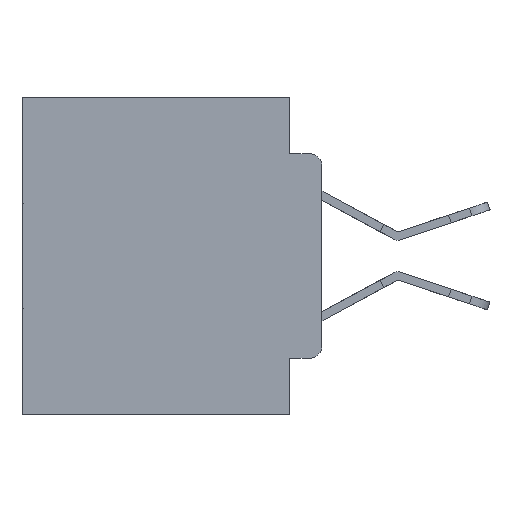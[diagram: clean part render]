
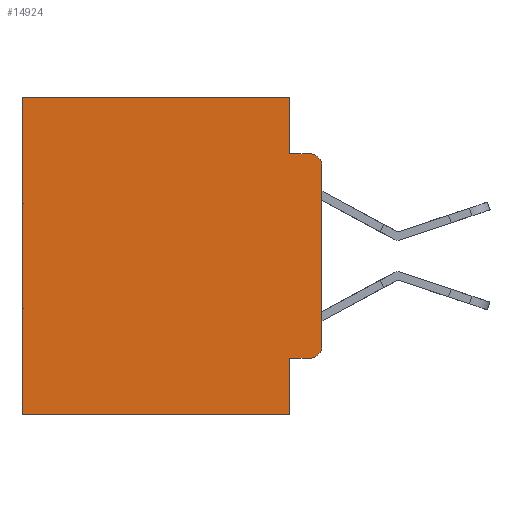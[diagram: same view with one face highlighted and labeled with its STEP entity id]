
A CAD part, left-side view. The second image highlights one B-rep face of the part: STEP entity #14924.
In plain terms, the highlighted planar face has unit normal (-1, 0, 0).
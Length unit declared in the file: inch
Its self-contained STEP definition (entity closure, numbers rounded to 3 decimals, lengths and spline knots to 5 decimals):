
#461 = DIRECTION ( 'NONE',  ( 0., -1., 0. ) ) ;
#847 = ORIENTED_EDGE ( 'NONE', *, *, #24118, .T. ) ;
#1697 = LINE ( 'NONE', #16504, #26920 ) ;
#1742 = LINE ( 'NONE', #30964, #8446 ) ;
#2425 = DIRECTION ( 'NONE',  ( -1., 0., 0. ) ) ;
#3101 = CARTESIAN_POINT ( 'NONE',  ( 0.298, 0., 0. ) ) ;
#3531 = VERTEX_POINT ( 'NONE', #8795 ) ;
#4022 = CARTESIAN_POINT ( 'NONE',  ( 0.298, 0.473, 0. ) ) ;
#4408 = ORIENTED_EDGE ( 'NONE', *, *, #8390, .F. ) ;
#4509 = EDGE_CURVE ( 'NONE', #24833, #29772, #18690, .T. ) ;
#4597 = CARTESIAN_POINT ( 'NONE',  ( 0.298, 0.02, -0.4115 ) ) ;
#4876 = CARTESIAN_POINT ( 'NONE',  ( 0.298, 0.051, 0. ) ) ;
#4918 = LINE ( 'NONE', #25913, #17300 ) ;
#5654 = DIRECTION ( 'NONE',  ( 0., 0., -1. ) ) ;
#5695 = VECTOR ( 'NONE', #27521, 39.37008 ) ;
#6582 = DIRECTION ( 'NONE',  ( 0., 0., -1. ) ) ;
#7586 = ORIENTED_EDGE ( 'NONE', *, *, #30619, .F. ) ;
#8390 = EDGE_CURVE ( 'NONE', #15049, #25976, #20808, .T. ) ;
#8446 = VECTOR ( 'NONE', #16836, 39.37008 ) ;
#8795 = CARTESIAN_POINT ( 'NONE',  ( 0.298, 0.051, -0.4115 ) ) ;
#9903 = ORIENTED_EDGE ( 'NONE', *, *, #19263, .T. ) ;
#9938 = CARTESIAN_POINT ( 'NONE',  ( 0.298, 0.473, -0.5 ) ) ;
#10428 = CARTESIAN_POINT ( 'NONE',  ( 0.298, 0.051, -0.5 ) ) ;
#10739 = VERTEX_POINT ( 'NONE', #20066 ) ;
#10905 = FACE_OUTER_BOUND ( 'NONE', #30051, .T. ) ;
#11100 = AXIS2_PLACEMENT_3D ( 'NONE', #3101, #20354, #5654 ) ;
#11311 = EDGE_CURVE ( 'NONE', #15049, #10739, #18377, .T. ) ;
#11324 = VECTOR ( 'NONE', #461, 39.37008 ) ;
#11823 = ORIENTED_EDGE ( 'NONE', *, *, #30928, .F. ) ;
#12268 = CARTESIAN_POINT ( 'NONE',  ( 0.298, 0.02, -0.3915 ) ) ;
#12626 = ORIENTED_EDGE ( 'NONE', *, *, #4509, .T. ) ;
#13394 = VERTEX_POINT ( 'NONE', #10428 ) ;
#14208 = EDGE_CURVE ( 'NONE', #3531, #27843, #17866, .T. ) ;
#14398 = VECTOR ( 'NONE', #19145, 39.37008 ) ;
#14539 = CARTESIAN_POINT ( 'NONE',  ( 0.298, 0.051, -0.0885 ) ) ;
#14729 = VECTOR ( 'NONE', #6582, 39.37008 ) ;
#14781 = DIRECTION ( 'NONE',  ( 0., 0., -1. ) ) ;
#14924 = ADVANCED_FACE ( 'NONE', ( #10905 ), #17952, .F. ) ;
#15049 = VERTEX_POINT ( 'NONE', #20870 ) ;
#15454 = CARTESIAN_POINT ( 'NONE',  ( 0.298, 0.051, -0.4115 ) ) ;
#15713 = ORIENTED_EDGE ( 'NONE', *, *, #14208, .T. ) ;
#15760 = AXIS2_PLACEMENT_3D ( 'NONE', #12268, #29025, #14781 ) ;
#16504 = CARTESIAN_POINT ( 'NONE',  ( 0.298, 0.051, 0. ) ) ;
#16836 = DIRECTION ( 'NONE',  ( 0., 1., 0. ) ) ;
#17300 = VECTOR ( 'NONE', #21159, 39.37008 ) ;
#17305 = CARTESIAN_POINT ( 'NONE',  ( 0.298, 0.02, -0.1085 ) ) ;
#17590 = ORIENTED_EDGE ( 'NONE', *, *, #11311, .T. ) ;
#17866 = LINE ( 'NONE', #15454, #11324 ) ;
#17952 = PLANE ( 'NONE',  #11100 ) ;
#18350 = ORIENTED_EDGE ( 'NONE', *, *, #30535, .F. ) ;
#18377 = CIRCLE ( 'NONE', #22260, 0.02 ) ;
#18480 = EDGE_CURVE ( 'NONE', #3531, #13394, #1697, .T. ) ;
#18690 = LINE ( 'NONE', #30323, #19447 ) ;
#18784 = LINE ( 'NONE', #22796, #5695 ) ;
#19145 = DIRECTION ( 'NONE',  ( 0., 0., -1. ) ) ;
#19263 = EDGE_CURVE ( 'NONE', #27843, #25976, #29083, .T. ) ;
#19447 = VECTOR ( 'NONE', #25054, 39.37008 ) ;
#19733 = DIRECTION ( 'NONE',  ( 0., 0., -1. ) ) ;
#20066 = CARTESIAN_POINT ( 'NONE',  ( 0.298, 0.02, -0.0885 ) ) ;
#20354 = DIRECTION ( 'NONE',  ( 1., 0., 0. ) ) ;
#20601 = ORIENTED_EDGE ( 'NONE', *, *, #18480, .F. ) ;
#20808 = LINE ( 'NONE', #28567, #14398 ) ;
#20870 = CARTESIAN_POINT ( 'NONE',  ( 0.298, 0., -0.1085 ) ) ;
#21159 = DIRECTION ( 'NONE',  ( 0., 0., -1. ) ) ;
#22260 = AXIS2_PLACEMENT_3D ( 'NONE', #17305, #2425, #19733 ) ;
#22796 = CARTESIAN_POINT ( 'NONE',  ( 0.298, 0.051, -0.0885 ) ) ;
#23073 = CARTESIAN_POINT ( 'NONE',  ( 0.298, 0.473, 0. ) ) ;
#24118 = EDGE_CURVE ( 'NONE', #29772, #30760, #25933, .T. ) ;
#24833 = VERTEX_POINT ( 'NONE', #4876 ) ;
#25054 = DIRECTION ( 'NONE',  ( 0., 1., 0. ) ) ;
#25913 = CARTESIAN_POINT ( 'NONE',  ( 0.298, 0.051, 0. ) ) ;
#25933 = LINE ( 'NONE', #4022, #14729 ) ;
#25976 = VERTEX_POINT ( 'NONE', #28896 ) ;
#26920 = VECTOR ( 'NONE', #30748, 39.37008 ) ;
#27521 = DIRECTION ( 'NONE',  ( 0., -1., 0. ) ) ;
#27843 = VERTEX_POINT ( 'NONE', #4597 ) ;
#28289 = VERTEX_POINT ( 'NONE', #14539 ) ;
#28567 = CARTESIAN_POINT ( 'NONE',  ( 0.298, 0., 0. ) ) ;
#28896 = CARTESIAN_POINT ( 'NONE',  ( 0.298, 0., -0.3915 ) ) ;
#29025 = DIRECTION ( 'NONE',  ( -1., 0., 0. ) ) ;
#29083 = CIRCLE ( 'NONE', #15760, 0.02 ) ;
#29772 = VERTEX_POINT ( 'NONE', #23073 ) ;
#30051 = EDGE_LOOP ( 'NONE', ( #4408, #17590, #11823, #18350, #12626, #847, #7586, #20601, #15713, #9903 ) ) ;
#30323 = CARTESIAN_POINT ( 'NONE',  ( 0.298, 0., 0. ) ) ;
#30535 = EDGE_CURVE ( 'NONE', #24833, #28289, #4918, .T. ) ;
#30619 = EDGE_CURVE ( 'NONE', #13394, #30760, #1742, .T. ) ;
#30748 = DIRECTION ( 'NONE',  ( 0., 0., -1. ) ) ;
#30760 = VERTEX_POINT ( 'NONE', #9938 ) ;
#30928 = EDGE_CURVE ( 'NONE', #28289, #10739, #18784, .T. ) ;
#30964 = CARTESIAN_POINT ( 'NONE',  ( 0.298, 0., -0.5 ) ) ;
